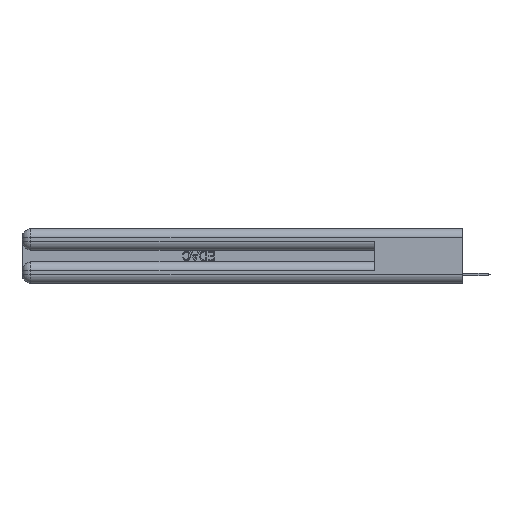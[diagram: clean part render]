
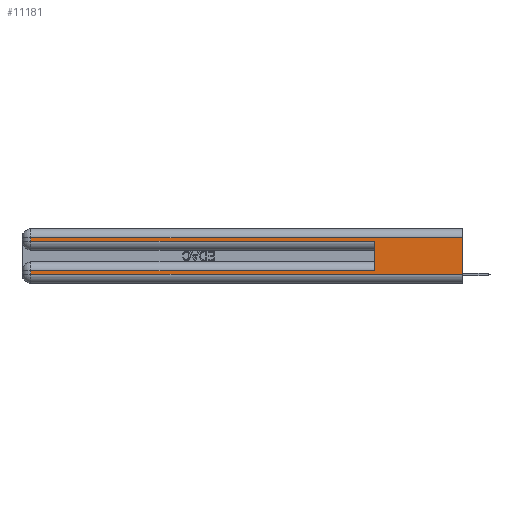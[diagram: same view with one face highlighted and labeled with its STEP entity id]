
A CAD part, left-side view. The second image highlights one B-rep face of the part: STEP entity #11181.
In plain terms, the highlighted planar face has unit normal (-1, 0, 0).
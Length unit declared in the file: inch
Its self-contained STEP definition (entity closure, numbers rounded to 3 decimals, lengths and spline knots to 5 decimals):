
#907 = CARTESIAN_POINT ( 'NONE',  ( 0., 2.94, 0.285 ) ) ;
#1080 = DIRECTION ( 'NONE',  ( 1., 0., 0. ) ) ;
#1359 = CARTESIAN_POINT ( 'NONE',  ( 0., 0.6, 0.145 ) ) ;
#1665 = VECTOR ( 'NONE', #6754, 39.37008 ) ;
#1761 = LINE ( 'NONE', #14633, #24868 ) ;
#2081 = EDGE_CURVE ( 'NONE', #2191, #31002, #11495, .T. ) ;
#2191 = VERTEX_POINT ( 'NONE', #13706 ) ;
#3132 = DIRECTION ( 'NONE',  ( 0., -1., 0. ) ) ;
#3381 = VECTOR ( 'NONE', #14975, 39.37008 ) ;
#3582 = VERTEX_POINT ( 'NONE', #20738 ) ;
#3808 = VECTOR ( 'NONE', #7197, 39.37008 ) ;
#5978 = CARTESIAN_POINT ( 'NONE',  ( 0., 2.94, 0.37 ) ) ;
#6105 = CARTESIAN_POINT ( 'NONE',  ( 0., 2.94, 0.06 ) ) ;
#6754 = DIRECTION ( 'NONE',  ( 0., 0., -1. ) ) ;
#7197 = DIRECTION ( 'NONE',  ( 0., -1., 0. ) ) ;
#7569 = LINE ( 'NONE', #24443, #3381 ) ;
#8335 = CARTESIAN_POINT ( 'NONE',  ( 0., 0.6, 0.285 ) ) ;
#8902 = VERTEX_POINT ( 'NONE', #25382 ) ;
#9816 = ORIENTED_EDGE ( 'NONE', *, *, #22047, .T. ) ;
#10096 = VERTEX_POINT ( 'NONE', #8335 ) ;
#10482 = VERTEX_POINT ( 'NONE', #907 ) ;
#11082 = CARTESIAN_POINT ( 'NONE',  ( 0., 0., 0.31 ) ) ;
#11181 = ADVANCED_FACE ( 'NONE', ( #26374 ), #29561, .F. ) ;
#11495 = LINE ( 'NONE', #24025, #19519 ) ;
#12180 = ORIENTED_EDGE ( 'NONE', *, *, #15029, .T. ) ;
#12318 = EDGE_CURVE ( 'NONE', #10482, #10096, #22846, .T. ) ;
#12580 = CARTESIAN_POINT ( 'NONE',  ( 0., 0., 0.285 ) ) ;
#12758 = ORIENTED_EDGE ( 'NONE', *, *, #25186, .F. ) ;
#12851 = ORIENTED_EDGE ( 'NONE', *, *, #24850, .T. ) ;
#13402 = CARTESIAN_POINT ( 'NONE',  ( 0., 0., 0.37 ) ) ;
#13706 = CARTESIAN_POINT ( 'NONE',  ( 0., 0., 0.31 ) ) ;
#14633 = CARTESIAN_POINT ( 'NONE',  ( 0., 2.94, 0.37 ) ) ;
#14676 = LINE ( 'NONE', #1359, #18895 ) ;
#14975 = DIRECTION ( 'NONE',  ( 0., 1., 0. ) ) ;
#15029 = EDGE_CURVE ( 'NONE', #8902, #3582, #7569, .T. ) ;
#15200 = VERTEX_POINT ( 'NONE', #6105 ) ;
#15661 = AXIS2_PLACEMENT_3D ( 'NONE', #13402, #1080, #20616 ) ;
#15985 = DIRECTION ( 'NONE',  ( 0., 1., 0. ) ) ;
#16666 = CARTESIAN_POINT ( 'NONE',  ( 0., 0., 0.06 ) ) ;
#16893 = LINE ( 'NONE', #11082, #26713 ) ;
#17083 = DIRECTION ( 'NONE',  ( 0., 0., -1. ) ) ;
#17133 = LINE ( 'NONE', #16666, #3808 ) ;
#17245 = VECTOR ( 'NONE', #3132, 39.37008 ) ;
#18895 = VECTOR ( 'NONE', #22527, 39.37008 ) ;
#19519 = VECTOR ( 'NONE', #23687, 39.37008 ) ;
#20616 = DIRECTION ( 'NONE',  ( 0., 0., -1. ) ) ;
#20738 = CARTESIAN_POINT ( 'NONE',  ( 0., 2.94, 0.085 ) ) ;
#20896 = ORIENTED_EDGE ( 'NONE', *, *, #2081, .F. ) ;
#22047 = EDGE_CURVE ( 'NONE', #15200, #31002, #17133, .T. ) ;
#22527 = DIRECTION ( 'NONE',  ( 0., 0., 1. ) ) ;
#22572 = ORIENTED_EDGE ( 'NONE', *, *, #12318, .T. ) ;
#22846 = LINE ( 'NONE', #12580, #17245 ) ;
#23687 = DIRECTION ( 'NONE',  ( 0., 0., -1. ) ) ;
#23879 = CARTESIAN_POINT ( 'NONE',  ( 0., 2.94, 0.31 ) ) ;
#24025 = CARTESIAN_POINT ( 'NONE',  ( 0., 0., 0.37 ) ) ;
#24443 = CARTESIAN_POINT ( 'NONE',  ( 0., 0., 0.085 ) ) ;
#24850 = EDGE_CURVE ( 'NONE', #24865, #10482, #1761, .T. ) ;
#24865 = VERTEX_POINT ( 'NONE', #23879 ) ;
#24868 = VECTOR ( 'NONE', #17083, 39.37008 ) ;
#25186 = EDGE_CURVE ( 'NONE', #8902, #10096, #14676, .T. ) ;
#25382 = CARTESIAN_POINT ( 'NONE',  ( 0., 0.6, 0.085 ) ) ;
#25892 = LINE ( 'NONE', #5978, #1665 ) ;
#26230 = EDGE_LOOP ( 'NONE', ( #20896, #30548, #12851, #22572, #12758, #12180, #29230, #9816 ) ) ;
#26374 = FACE_OUTER_BOUND ( 'NONE', #26230, .T. ) ;
#26713 = VECTOR ( 'NONE', #15985, 39.37008 ) ;
#29230 = ORIENTED_EDGE ( 'NONE', *, *, #31363, .T. ) ;
#29561 = PLANE ( 'NONE',  #15661 ) ;
#30539 = EDGE_CURVE ( 'NONE', #2191, #24865, #16893, .T. ) ;
#30548 = ORIENTED_EDGE ( 'NONE', *, *, #30539, .T. ) ;
#31002 = VERTEX_POINT ( 'NONE', #31127 ) ;
#31127 = CARTESIAN_POINT ( 'NONE',  ( 0., 0., 0.06 ) ) ;
#31363 = EDGE_CURVE ( 'NONE', #3582, #15200, #25892, .T. ) ;
